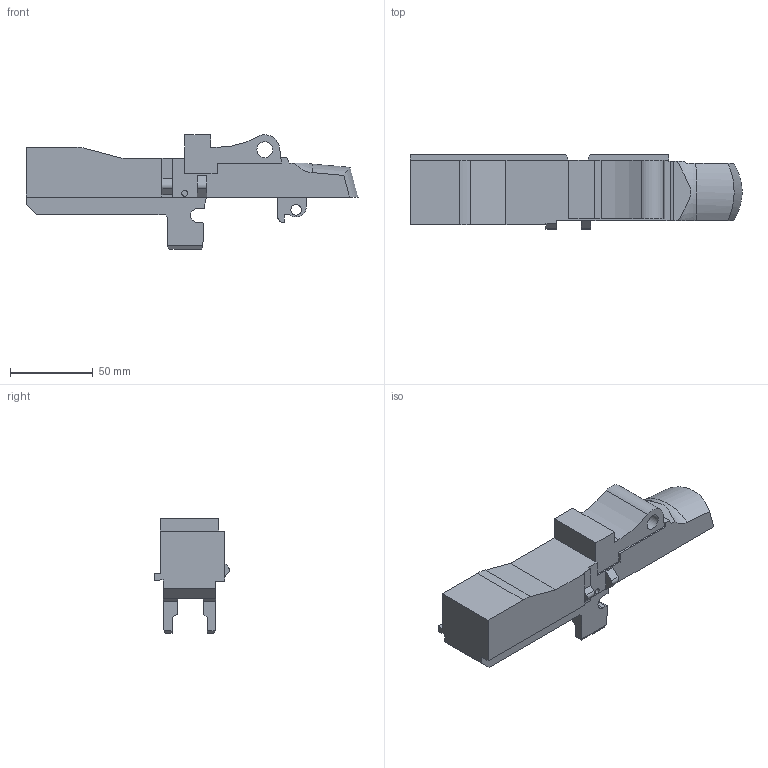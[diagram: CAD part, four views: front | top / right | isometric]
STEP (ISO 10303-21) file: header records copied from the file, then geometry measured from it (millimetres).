
FILE_DESCRIPTION(('STEP AP214'),'1');
FILE_NAME('M14Reciever.stp','2016-06-08T19:15:39',('DanielL'),('None'),'Spatial InterOp 3D','Cimatron E 12.0',' ');
FILE_SCHEMA(('automotive_design'));
Length unit declared in the file: inch
Products named in the file (1): 1
Bounding box: 200.91 x 45.17 x 69.24 mm (x, y, z)
Volume: 239475.8 mm3; surface area: 36540.4 mm2
Topology: 1 solids, 1 shells, 112 faces, 325 edges, 216 vertices
Faces by surface type: plane 94, cylinder 16, torus 1, bspline 1
Full cylindrical faces by diameter (mm): 3.543 x1, 6.388 x1, 6.426 x1, 9.55 x1
Entity records: 6264 total; most frequent: CARTESIAN_POINT 789, ORIENTED_EDGE 638, DIRECTION 573, STYLED_ITEM 432, PRESENTATION_STYLE_ASSIGNMENT 432, COLOUR_RGB 432, EDGE_CURVE 319, CURVE_STYLE 319
